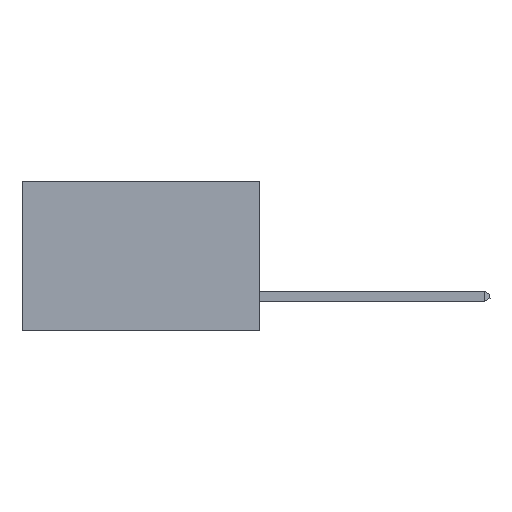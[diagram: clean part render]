
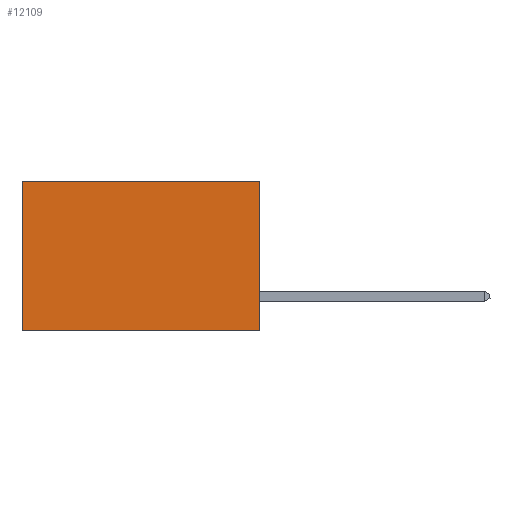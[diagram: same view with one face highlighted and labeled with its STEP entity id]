
A CAD part, left-side view. The second image highlights one B-rep face of the part: STEP entity #12109.
In plain terms, the highlighted planar face has unit normal (-1, 0, 0).
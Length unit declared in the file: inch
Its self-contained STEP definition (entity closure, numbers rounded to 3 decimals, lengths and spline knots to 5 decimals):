
#124 = LINE ( 'NONE', #802, #5380 ) ;
#470 = VERTEX_POINT ( 'NONE', #11848 ) ;
#524 = DIRECTION ( 'NONE',  ( 0., 1., 0. ) ) ;
#802 = CARTESIAN_POINT ( 'NONE',  ( 0.277, 0., 0. ) ) ;
#858 = ORIENTED_EDGE ( 'NONE', *, *, #11413, .T. ) ;
#1051 = DIRECTION ( 'NONE',  ( 1., 0., 0. ) ) ;
#1418 = VECTOR ( 'NONE', #1713, 39.37008 ) ;
#1713 = DIRECTION ( 'NONE',  ( 0., 1., 0. ) ) ;
#1961 = VERTEX_POINT ( 'NONE', #9859 ) ;
#2094 = EDGE_CURVE ( 'NONE', #1961, #9695, #4021, .T. ) ;
#2244 = LINE ( 'NONE', #10455, #4523 ) ;
#3208 = CARTESIAN_POINT ( 'NONE',  ( 0.277, 0., -0.37 ) ) ;
#3544 = EDGE_CURVE ( 'NONE', #470, #7727, #124, .T. ) ;
#4021 = LINE ( 'NONE', #12094, #1418 ) ;
#4240 = ORIENTED_EDGE ( 'NONE', *, *, #8385, .F. ) ;
#4523 = VECTOR ( 'NONE', #11342, 39.37008 ) ;
#5178 = CARTESIAN_POINT ( 'NONE',  ( 0.277, 0.59, 0. ) ) ;
#5238 = DIRECTION ( 'NONE',  ( 0., 0., -1. ) ) ;
#5380 = VECTOR ( 'NONE', #524, 39.37008 ) ;
#5488 = ORIENTED_EDGE ( 'NONE', *, *, #3544, .T. ) ;
#6900 = PLANE ( 'NONE',  #11139 ) ;
#7365 = VECTOR ( 'NONE', #5238, 39.37008 ) ;
#7727 = VERTEX_POINT ( 'NONE', #5178 ) ;
#7834 = DIRECTION ( 'NONE',  ( 0., 0., -1. ) ) ;
#7942 = FACE_OUTER_BOUND ( 'NONE', #9722, .T. ) ;
#7990 = ORIENTED_EDGE ( 'NONE', *, *, #2094, .F. ) ;
#8385 = EDGE_CURVE ( 'NONE', #470, #1961, #12173, .T. ) ;
#8738 = CARTESIAN_POINT ( 'NONE',  ( 0.277, 0., -0.37 ) ) ;
#9695 = VERTEX_POINT ( 'NONE', #11855 ) ;
#9722 = EDGE_LOOP ( 'NONE', ( #858, #7990, #4240, #5488 ) ) ;
#9859 = CARTESIAN_POINT ( 'NONE',  ( 0.277, 0., -0.37 ) ) ;
#10455 = CARTESIAN_POINT ( 'NONE',  ( 0.277, 0.59, -0.37 ) ) ;
#11139 = AXIS2_PLACEMENT_3D ( 'NONE', #8738, #1051, #7834 ) ;
#11342 = DIRECTION ( 'NONE',  ( 0., 0., -1. ) ) ;
#11413 = EDGE_CURVE ( 'NONE', #7727, #9695, #2244, .T. ) ;
#11848 = CARTESIAN_POINT ( 'NONE',  ( 0.277, 0., 0. ) ) ;
#11855 = CARTESIAN_POINT ( 'NONE',  ( 0.277, 0.59, -0.37 ) ) ;
#12094 = CARTESIAN_POINT ( 'NONE',  ( 0.277, 0., -0.37 ) ) ;
#12109 = ADVANCED_FACE ( 'NONE', ( #7942 ), #6900, .F. ) ;
#12173 = LINE ( 'NONE', #3208, #7365 ) ;
